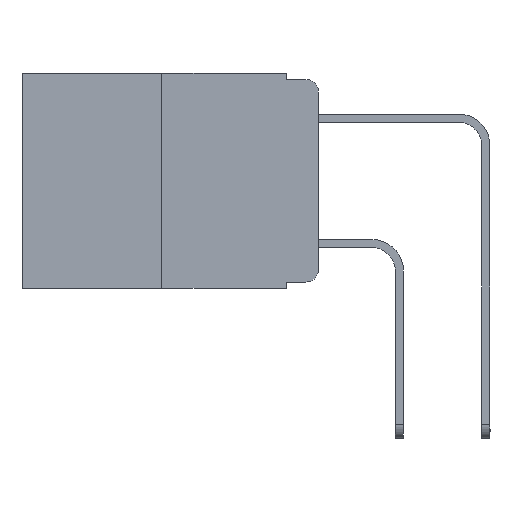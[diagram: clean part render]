
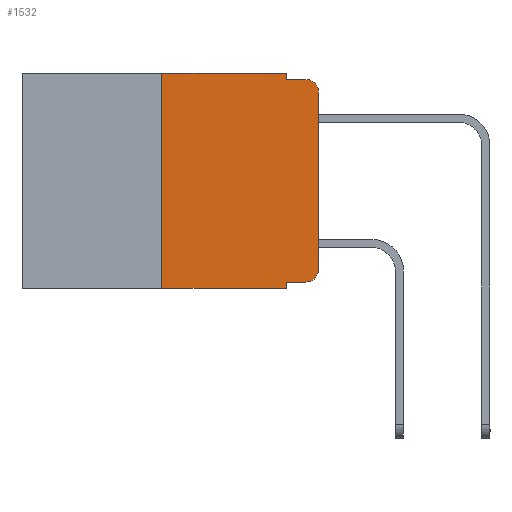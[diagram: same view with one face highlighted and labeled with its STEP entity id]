
A CAD part, left-side view. The second image highlights one B-rep face of the part: STEP entity #1532.
In plain terms, the highlighted planar face has unit normal (-1, 0, 0).
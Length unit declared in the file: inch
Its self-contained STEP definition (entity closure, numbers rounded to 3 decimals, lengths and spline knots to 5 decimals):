
#199 = VECTOR ( 'NONE', #9078, 39.37008 ) ;
#313 = CARTESIAN_POINT ( 'NONE',  ( 0., 0.02, -0.03 ) ) ;
#325 = CARTESIAN_POINT ( 'NONE',  ( 0., 0., -0.313 ) ) ;
#546 = CARTESIAN_POINT ( 'NONE',  ( 0., 0.02, -0.333 ) ) ;
#626 = VECTOR ( 'NONE', #8753, 39.37008 ) ;
#712 = EDGE_CURVE ( 'NONE', #2985, #4969, #10288, .T. ) ;
#771 = DIRECTION ( 'NONE',  ( -1., 0., 0. ) ) ;
#811 = CARTESIAN_POINT ( 'NONE',  ( 0., 0.473, -0.343 ) ) ;
#954 = CARTESIAN_POINT ( 'NONE',  ( 0., 0.25, -0.343 ) ) ;
#1063 = CARTESIAN_POINT ( 'NONE',  ( 0., 0.051, 0. ) ) ;
#1155 = EDGE_CURVE ( 'NONE', #4055, #11223, #3199, .T. ) ;
#1418 = LINE ( 'NONE', #811, #199 ) ;
#1485 = CIRCLE ( 'NONE', #3711, 0.02 ) ;
#1532 = ADVANCED_FACE ( 'NONE', ( #3981 ), #3344, .F. ) ;
#2093 = CARTESIAN_POINT ( 'NONE',  ( 0., 0.051, 0. ) ) ;
#2120 = VECTOR ( 'NONE', #7053, 39.37008 ) ;
#2128 = EDGE_CURVE ( 'NONE', #10134, #4969, #1485, .T. ) ;
#2342 = CIRCLE ( 'NONE', #4224, 0.02 ) ;
#2449 = CARTESIAN_POINT ( 'NONE',  ( 0., 0., -0.03 ) ) ;
#2599 = CARTESIAN_POINT ( 'NONE',  ( 0., 0.051, -0.333 ) ) ;
#2659 = DIRECTION ( 'NONE',  ( 0., 0., -1. ) ) ;
#2810 = VECTOR ( 'NONE', #4131, 39.37008 ) ;
#2898 = CARTESIAN_POINT ( 'NONE',  ( 0., 0.051, 0. ) ) ;
#2980 = EDGE_CURVE ( 'NONE', #8296, #8022, #1418, .T. ) ;
#2985 = VERTEX_POINT ( 'NONE', #5476 ) ;
#3199 = LINE ( 'NONE', #5893, #2120 ) ;
#3308 = DIRECTION ( 'NONE',  ( 0., 0., -1. ) ) ;
#3344 = PLANE ( 'NONE',  #3777 ) ;
#3711 = AXIS2_PLACEMENT_3D ( 'NONE', #313, #5397, #3715 ) ;
#3715 = DIRECTION ( 'NONE',  ( 0., 0., -1. ) ) ;
#3777 = AXIS2_PLACEMENT_3D ( 'NONE', #6846, #4133, #3308 ) ;
#3853 = VERTEX_POINT ( 'NONE', #325 ) ;
#3981 = FACE_OUTER_BOUND ( 'NONE', #4815, .T. ) ;
#4032 = ORIENTED_EDGE ( 'NONE', *, *, #9083, .F. ) ;
#4055 = VERTEX_POINT ( 'NONE', #8362 ) ;
#4131 = DIRECTION ( 'NONE',  ( 0., 0., 1. ) ) ;
#4133 = DIRECTION ( 'NONE',  ( 1., 0., 0. ) ) ;
#4224 = AXIS2_PLACEMENT_3D ( 'NONE', #5929, #771, #2659 ) ;
#4392 = DIRECTION ( 'NONE',  ( 0., -1., 0. ) ) ;
#4444 = CARTESIAN_POINT ( 'NONE',  ( 0., 0.051, -0.343 ) ) ;
#4667 = ORIENTED_EDGE ( 'NONE', *, *, #8853, .T. ) ;
#4716 = EDGE_CURVE ( 'NONE', #9257, #3853, #2342, .T. ) ;
#4815 = EDGE_LOOP ( 'NONE', ( #10823, #8790, #10825, #7964, #8430, #7260, #10110, #4032, #4667, #5489 ) ) ;
#4969 = VERTEX_POINT ( 'NONE', #10582 ) ;
#5008 = VECTOR ( 'NONE', #11144, 39.37008 ) ;
#5374 = EDGE_CURVE ( 'NONE', #11223, #2985, #5750, .T. ) ;
#5397 = DIRECTION ( 'NONE',  ( -1., 0., 0. ) ) ;
#5476 = CARTESIAN_POINT ( 'NONE',  ( 0., 0.051, -0.01 ) ) ;
#5489 = ORIENTED_EDGE ( 'NONE', *, *, #4716, .T. ) ;
#5750 = LINE ( 'NONE', #1063, #626 ) ;
#5822 = LINE ( 'NONE', #2599, #5008 ) ;
#5893 = CARTESIAN_POINT ( 'NONE',  ( 0., 0.473, 0. ) ) ;
#5929 = CARTESIAN_POINT ( 'NONE',  ( 0., 0.02, -0.313 ) ) ;
#6518 = VECTOR ( 'NONE', #7154, 39.37008 ) ;
#6625 = VERTEX_POINT ( 'NONE', #9242 ) ;
#6846 = CARTESIAN_POINT ( 'NONE',  ( 0., 0.473, 0. ) ) ;
#7053 = DIRECTION ( 'NONE',  ( 0., -1., 0. ) ) ;
#7070 = LINE ( 'NONE', #2093, #6518 ) ;
#7154 = DIRECTION ( 'NONE',  ( 0., 0., -1. ) ) ;
#7260 = ORIENTED_EDGE ( 'NONE', *, *, #8950, .F. ) ;
#7964 = ORIENTED_EDGE ( 'NONE', *, *, #5374, .F. ) ;
#8022 = VERTEX_POINT ( 'NONE', #4444 ) ;
#8244 = VECTOR ( 'NONE', #4392, 39.37008 ) ;
#8296 = VERTEX_POINT ( 'NONE', #954 ) ;
#8362 = CARTESIAN_POINT ( 'NONE',  ( 0., 0.25, 0. ) ) ;
#8430 = ORIENTED_EDGE ( 'NONE', *, *, #1155, .F. ) ;
#8674 = EDGE_CURVE ( 'NONE', #3853, #10134, #10559, .T. ) ;
#8708 = CARTESIAN_POINT ( 'NONE',  ( 0., 0.25, 0. ) ) ;
#8753 = DIRECTION ( 'NONE',  ( 0., 0., -1. ) ) ;
#8790 = ORIENTED_EDGE ( 'NONE', *, *, #2128, .T. ) ;
#8853 = EDGE_CURVE ( 'NONE', #6625, #9257, #5822, .T. ) ;
#8950 = EDGE_CURVE ( 'NONE', #8296, #4055, #10885, .T. ) ;
#9071 = CARTESIAN_POINT ( 'NONE',  ( 0., 0., 0. ) ) ;
#9078 = DIRECTION ( 'NONE',  ( 0., -1., 0. ) ) ;
#9083 = EDGE_CURVE ( 'NONE', #6625, #8022, #7070, .T. ) ;
#9242 = CARTESIAN_POINT ( 'NONE',  ( 0., 0.051, -0.333 ) ) ;
#9257 = VERTEX_POINT ( 'NONE', #546 ) ;
#9650 = CARTESIAN_POINT ( 'NONE',  ( 0., 0.051, -0.01 ) ) ;
#10110 = ORIENTED_EDGE ( 'NONE', *, *, #2980, .T. ) ;
#10134 = VERTEX_POINT ( 'NONE', #2449 ) ;
#10288 = LINE ( 'NONE', #9650, #8244 ) ;
#10334 = VECTOR ( 'NONE', #10572, 39.37008 ) ;
#10559 = LINE ( 'NONE', #9071, #2810 ) ;
#10572 = DIRECTION ( 'NONE',  ( 0., 0., 1. ) ) ;
#10582 = CARTESIAN_POINT ( 'NONE',  ( 0., 0.02, -0.01 ) ) ;
#10823 = ORIENTED_EDGE ( 'NONE', *, *, #8674, .T. ) ;
#10825 = ORIENTED_EDGE ( 'NONE', *, *, #712, .F. ) ;
#10885 = LINE ( 'NONE', #8708, #10334 ) ;
#11144 = DIRECTION ( 'NONE',  ( 0., -1., 0. ) ) ;
#11223 = VERTEX_POINT ( 'NONE', #2898 ) ;
